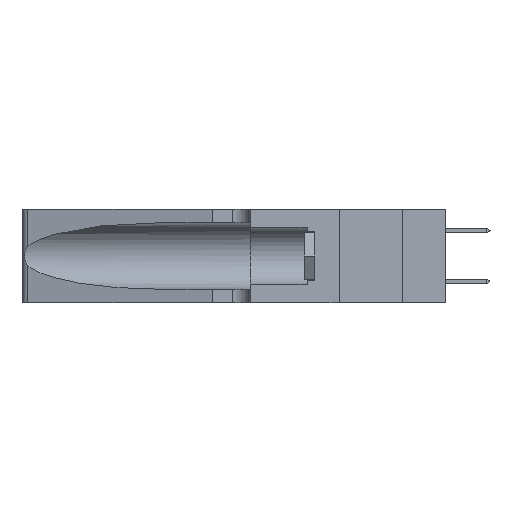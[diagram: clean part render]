
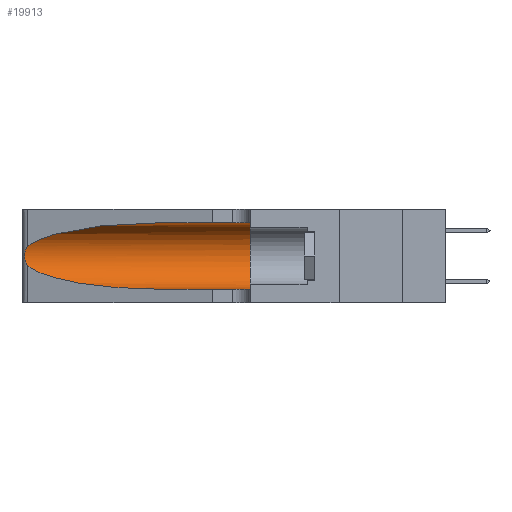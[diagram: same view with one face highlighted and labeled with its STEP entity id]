
A CAD part, left-side view. The second image highlights one B-rep face of the part: STEP entity #19913.
In plain terms, the highlighted cylindrical face has radius 3.308 mm (diameter 6.617 mm), a partial arc.
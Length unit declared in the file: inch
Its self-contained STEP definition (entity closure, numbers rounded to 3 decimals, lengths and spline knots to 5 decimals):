
#382 =( BOUNDED_CURVE ( )  B_SPLINE_CURVE ( 3, ( #8970, #383, #2533, #5128 ),
 .UNSPECIFIED., .F., .F. ) 
 B_SPLINE_CURVE_WITH_KNOTS ( ( 4, 4 ),
 ( 3.44316, 4.71239 ),
 .UNSPECIFIED. ) 
 CURVE ( )  GEOMETRIC_REPRESENTATION_ITEM ( )  RATIONAL_B_SPLINE_CURVE ( ( 1., 0.87, 0.87, 1. ) ) 
 REPRESENTATION_ITEM ( '' )  );
#383 = CARTESIAN_POINT ( 'NONE',  ( 0.2373, 1.15595, 0.08982 ) ) ;
#2220 = CARTESIAN_POINT ( 'NONE',  ( 0.1305, 1.61858, 0.05475 ) ) ;
#2533 = CARTESIAN_POINT ( 'NONE',  ( 0.18966, 0.96281, 0.05475 ) ) ;
#3405 = CARTESIAN_POINT ( 'NONE',  ( 0.18966, 0.96281, 0.31525 ) ) ;
#3597 = DIRECTION ( 'NONE',  ( 0., 0., 1. ) ) ;
#3937 = EDGE_LOOP ( 'NONE', ( #12665, #12519, #23683, #29906, #7765, #26614 ) ) ;
#3993 = VERTEX_POINT ( 'NONE', #30791 ) ;
#4068 = CARTESIAN_POINT ( 'NONE',  ( 0.25487, 1.22718, 0.22369 ) ) ;
#4468 = LINE ( 'NONE', #6646, #7482 ) ;
#4540 = EDGE_CURVE ( 'NONE', #3993, #6691, #4468, .T. ) ;
#4825 = EDGE_CURVE ( 'NONE', #29006, #18161, #25420, .T. ) ;
#5086 = CIRCLE ( 'NONE', #9318, 0.13025 ) ;
#5128 = CARTESIAN_POINT ( 'NONE',  ( 0.1305, 0.72297, 0.05475 ) ) ;
#6646 = CARTESIAN_POINT ( 'NONE',  ( 0.1305, 1.61858, 0.31525 ) ) ;
#6691 = VERTEX_POINT ( 'NONE', #14431 ) ;
#7374 = DIRECTION ( 'NONE',  ( 0., 0., -1. ) ) ;
#7482 = VECTOR ( 'NONE', #25776, 39.37008 ) ;
#7765 = ORIENTED_EDGE ( 'NONE', *, *, #28195, .F. ) ;
#7818 = FACE_OUTER_BOUND ( 'NONE', #3937, .T. ) ;
#8586 = CARTESIAN_POINT ( 'NONE',  ( 0.25555, 1.22994, 0.2215 ) ) ;
#8694 = CARTESIAN_POINT ( 'NONE',  ( 0.26075, 1.23896, 0.178 ) ) ;
#8970 = CARTESIAN_POINT ( 'NONE',  ( 0.25487, 1.22718, 0.14631 ) ) ;
#9318 = AXIS2_PLACEMENT_3D ( 'NONE', #27299, #17811, #3597 ) ;
#9447 = VERTEX_POINT ( 'NONE', #13500 ) ;
#9960 = EDGE_CURVE ( 'NONE', #9447, #18914, #16409, .T. ) ;
#10616 = CARTESIAN_POINT ( 'NONE',  ( 0.25487, 1.22718, 0.22369 ) ) ;
#12519 = ORIENTED_EDGE ( 'NONE', *, *, #9960, .T. ) ;
#12665 = ORIENTED_EDGE ( 'NONE', *, *, #22172, .T. ) ;
#13375 = CARTESIAN_POINT ( 'NONE',  ( 0.25639, 1.23184, 0.21858 ) ) ;
#13500 = CARTESIAN_POINT ( 'NONE',  ( 0.25487, 1.22718, 0.22369 ) ) ;
#14431 = CARTESIAN_POINT ( 'NONE',  ( 0.1305, 0.35, 0.31525 ) ) ;
#14540 = VECTOR ( 'NONE', #23909, 39.37008 ) ;
#14628 = CARTESIAN_POINT ( 'NONE',  ( 0.1305, 0.35, 0.05475 ) ) ;
#15672 = CARTESIAN_POINT ( 'NONE',  ( 0.25555, 1.22993, 0.14849 ) ) ;
#15879 = CARTESIAN_POINT ( 'NONE',  ( 0.26018, 1.23835, 0.19895 ) ) ;
#16409 = B_SPLINE_CURVE_WITH_KNOTS ( 'NONE', 3,
 ( #4068, #8586, #13375, #25617, #23194, #15879, #20801, #8694, #18077, #27778, #23295, #27985, #15672, #30381 ),
 .UNSPECIFIED., .F., .F.,
 ( 4, 2, 2, 2, 2, 2, 4 ),
 ( 0., 0.00027, 0.00053, 0.00107, 0.0016, 0.00187, 0.00214 ),
 .UNSPECIFIED. ) ;
#16547 = DIRECTION ( 'NONE',  ( 0., -1., 0. ) ) ;
#17778 = CARTESIAN_POINT ( 'NONE',  ( 0.25487, 1.22718, 0.14631 ) ) ;
#17811 = DIRECTION ( 'NONE',  ( 0., 1., 0. ) ) ;
#17919 = CYLINDRICAL_SURFACE ( 'NONE', #21995, 0.13025 ) ;
#18077 = CARTESIAN_POINT ( 'NONE',  ( 0.26017, 1.23833, 0.17102 ) ) ;
#18161 = VERTEX_POINT ( 'NONE', #14628 ) ;
#18174 = EDGE_CURVE ( 'NONE', #18914, #29006, #382, .T. ) ;
#18914 = VERTEX_POINT ( 'NONE', #17778 ) ;
#19173 = CARTESIAN_POINT ( 'NONE',  ( 0.1305, 1.61858, 0.185 ) ) ;
#19913 = ADVANCED_FACE ( 'NONE', ( #7818 ), #17919, .F. ) ;
#20030 = CARTESIAN_POINT ( 'NONE',  ( 0.2373, 1.15595, 0.28018 ) ) ;
#20801 = CARTESIAN_POINT ( 'NONE',  ( 0.26075, 1.23896, 0.19203 ) ) ;
#21995 = AXIS2_PLACEMENT_3D ( 'NONE', #19173, #16547, #7374 ) ;
#22172 = EDGE_CURVE ( 'NONE', #3993, #9447, #26192, .T. ) ;
#22305 = CARTESIAN_POINT ( 'NONE',  ( 0.1305, 0.72297, 0.31525 ) ) ;
#23194 = CARTESIAN_POINT ( 'NONE',  ( 0.25854, 1.2359, 0.20912 ) ) ;
#23295 = CARTESIAN_POINT ( 'NONE',  ( 0.25789, 1.23486, 0.15765 ) ) ;
#23683 = ORIENTED_EDGE ( 'NONE', *, *, #18174, .T. ) ;
#23909 = DIRECTION ( 'NONE',  ( 0., -1., 0. ) ) ;
#25420 = LINE ( 'NONE', #2220, #14540 ) ;
#25617 = CARTESIAN_POINT ( 'NONE',  ( 0.25787, 1.23484, 0.2124 ) ) ;
#25776 = DIRECTION ( 'NONE',  ( 0., -1., 0. ) ) ;
#26192 =( BOUNDED_CURVE ( )  B_SPLINE_CURVE ( 3, ( #22305, #3405, #20030, #10616 ),
 .UNSPECIFIED., .F., .F. ) 
 B_SPLINE_CURVE_WITH_KNOTS ( ( 4, 4 ),
 ( 1.5708, 2.84003 ),
 .UNSPECIFIED. ) 
 CURVE ( )  GEOMETRIC_REPRESENTATION_ITEM ( )  RATIONAL_B_SPLINE_CURVE ( ( 1., 0.87, 0.87, 1. ) ) 
 REPRESENTATION_ITEM ( '' )  );
#26614 = ORIENTED_EDGE ( 'NONE', *, *, #4540, .F. ) ;
#27299 = CARTESIAN_POINT ( 'NONE',  ( 0.1305, 0.35, 0.185 ) ) ;
#27778 = CARTESIAN_POINT ( 'NONE',  ( 0.25856, 1.23593, 0.16098 ) ) ;
#27985 = CARTESIAN_POINT ( 'NONE',  ( 0.25639, 1.23186, 0.15144 ) ) ;
#28175 = CARTESIAN_POINT ( 'NONE',  ( 0.1305, 0.72297, 0.05475 ) ) ;
#28195 = EDGE_CURVE ( 'NONE', #6691, #18161, #5086, .T. ) ;
#29006 = VERTEX_POINT ( 'NONE', #28175 ) ;
#29906 = ORIENTED_EDGE ( 'NONE', *, *, #4825, .T. ) ;
#30381 = CARTESIAN_POINT ( 'NONE',  ( 0.25487, 1.22718, 0.14631 ) ) ;
#30791 = CARTESIAN_POINT ( 'NONE',  ( 0.1305, 0.72297, 0.31525 ) ) ;
